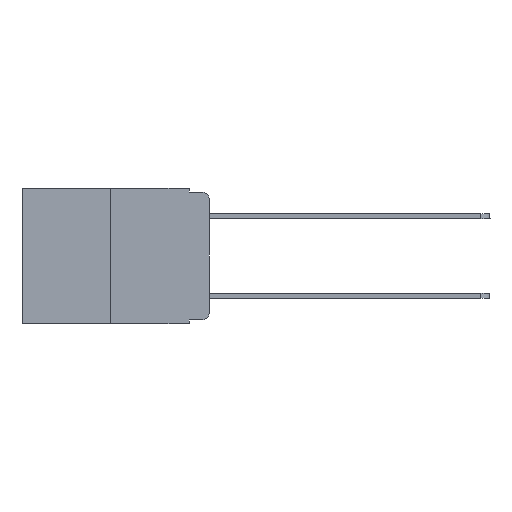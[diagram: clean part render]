
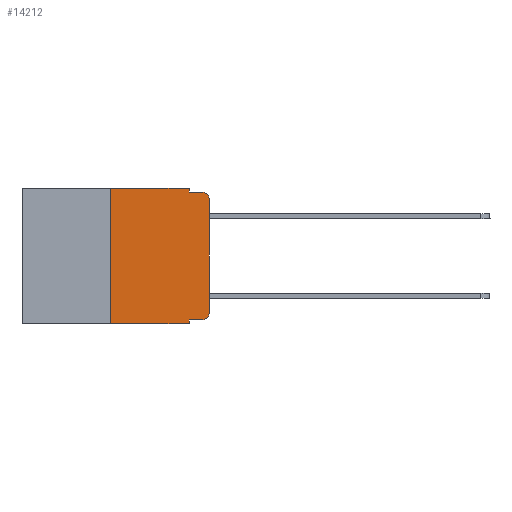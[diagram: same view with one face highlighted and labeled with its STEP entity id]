
A CAD part, left-side view. The second image highlights one B-rep face of the part: STEP entity #14212.
In plain terms, the highlighted planar face has unit normal (-1, 0, 0).
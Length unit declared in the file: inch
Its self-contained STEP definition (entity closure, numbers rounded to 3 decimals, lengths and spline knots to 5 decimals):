
#417 = DIRECTION ( 'NONE',  ( 0., -1., 0. ) ) ;
#524 = CARTESIAN_POINT ( 'NONE',  ( 0., 0.473, -0.343 ) ) ;
#1073 = CARTESIAN_POINT ( 'NONE',  ( 0., 0.051, -0.333 ) ) ;
#1278 = FACE_OUTER_BOUND ( 'NONE', #17155, .T. ) ;
#1283 = LINE ( 'NONE', #1073, #13073 ) ;
#1599 = CARTESIAN_POINT ( 'NONE',  ( 0., 0.051, 0. ) ) ;
#1648 = VECTOR ( 'NONE', #417, 39.37008 ) ;
#1770 = AXIS2_PLACEMENT_3D ( 'NONE', #12779, #19868, #8345 ) ;
#2055 = DIRECTION ( 'NONE',  ( -1., 0., 0. ) ) ;
#2143 = LINE ( 'NONE', #524, #1648 ) ;
#2580 = VERTEX_POINT ( 'NONE', #17380 ) ;
#4154 = CARTESIAN_POINT ( 'NONE',  ( 0., 0.051, 0. ) ) ;
#4368 = ORIENTED_EDGE ( 'NONE', *, *, #5768, .F. ) ;
#4468 = CARTESIAN_POINT ( 'NONE',  ( 0., 0.051, -0.333 ) ) ;
#4494 = CARTESIAN_POINT ( 'NONE',  ( 0., 0.02, -0.01 ) ) ;
#4663 = CARTESIAN_POINT ( 'NONE',  ( 0., 0., -0.03 ) ) ;
#4800 = VECTOR ( 'NONE', #13725, 39.37008 ) ;
#5119 = DIRECTION ( 'NONE',  ( 0., 0., -1. ) ) ;
#5168 = CARTESIAN_POINT ( 'NONE',  ( 0., 0.25, -0.343 ) ) ;
#5503 = CARTESIAN_POINT ( 'NONE',  ( 0., 0.02, -0.313 ) ) ;
#5768 = EDGE_CURVE ( 'NONE', #2580, #7699, #9974, .T. ) ;
#6413 = EDGE_CURVE ( 'NONE', #14480, #19937, #15610, .T. ) ;
#6715 = ORIENTED_EDGE ( 'NONE', *, *, #7337, .F. ) ;
#6822 = ORIENTED_EDGE ( 'NONE', *, *, #6413, .T. ) ;
#6877 = CARTESIAN_POINT ( 'NONE',  ( 0., 0.02, -0.03 ) ) ;
#7066 = AXIS2_PLACEMENT_3D ( 'NONE', #6877, #2055, #11632 ) ;
#7229 = VECTOR ( 'NONE', #16771, 39.37008 ) ;
#7337 = EDGE_CURVE ( 'NONE', #7699, #12888, #12559, .T. ) ;
#7699 = VERTEX_POINT ( 'NONE', #12933 ) ;
#7700 = VECTOR ( 'NONE', #20775, 39.37008 ) ;
#7811 = PLANE ( 'NONE',  #1770 ) ;
#7933 = VERTEX_POINT ( 'NONE', #9357 ) ;
#8112 = DIRECTION ( 'NONE',  ( 0., -1., 0. ) ) ;
#8345 = DIRECTION ( 'NONE',  ( 0., 0., -1. ) ) ;
#9282 = ORIENTED_EDGE ( 'NONE', *, *, #15526, .T. ) ;
#9315 = EDGE_CURVE ( 'NONE', #19937, #12888, #9506, .T. ) ;
#9357 = CARTESIAN_POINT ( 'NONE',  ( 0., 0.051, -0.343 ) ) ;
#9506 = CIRCLE ( 'NONE', #7066, 0.02 ) ;
#9676 = CIRCLE ( 'NONE', #19290, 0.02 ) ;
#9974 = LINE ( 'NONE', #1599, #19733 ) ;
#10031 = VERTEX_POINT ( 'NONE', #12865 ) ;
#10699 = CARTESIAN_POINT ( 'NONE',  ( 0., 0., -0.313 ) ) ;
#10761 = VERTEX_POINT ( 'NONE', #5168 ) ;
#10933 = ORIENTED_EDGE ( 'NONE', *, *, #13773, .F. ) ;
#11137 = EDGE_CURVE ( 'NONE', #10761, #7933, #2143, .T. ) ;
#11632 = DIRECTION ( 'NONE',  ( 0., 0., -1. ) ) ;
#11666 = CARTESIAN_POINT ( 'NONE',  ( 0., 0.25, 0. ) ) ;
#12178 = DIRECTION ( 'NONE',  ( -1., 0., 0. ) ) ;
#12559 = LINE ( 'NONE', #19217, #20457 ) ;
#12779 = CARTESIAN_POINT ( 'NONE',  ( 0., 0.473, 0. ) ) ;
#12865 = CARTESIAN_POINT ( 'NONE',  ( 0., 0.02, -0.333 ) ) ;
#12888 = VERTEX_POINT ( 'NONE', #4494 ) ;
#12933 = CARTESIAN_POINT ( 'NONE',  ( 0., 0.051, -0.01 ) ) ;
#13041 = ORIENTED_EDGE ( 'NONE', *, *, #17055, .F. ) ;
#13052 = LINE ( 'NONE', #11666, #19293 ) ;
#13073 = VECTOR ( 'NONE', #14188, 39.37008 ) ;
#13725 = DIRECTION ( 'NONE',  ( 0., 0., -1. ) ) ;
#13773 = EDGE_CURVE ( 'NONE', #15794, #2580, #14411, .T. ) ;
#14188 = DIRECTION ( 'NONE',  ( 0., -1., 0. ) ) ;
#14212 = ADVANCED_FACE ( 'NONE', ( #1278 ), #7811, .F. ) ;
#14217 = CARTESIAN_POINT ( 'NONE',  ( 0., 0., 0. ) ) ;
#14411 = LINE ( 'NONE', #16344, #7229 ) ;
#14480 = VERTEX_POINT ( 'NONE', #10699 ) ;
#15218 = ORIENTED_EDGE ( 'NONE', *, *, #16032, .F. ) ;
#15356 = ORIENTED_EDGE ( 'NONE', *, *, #9315, .T. ) ;
#15526 = EDGE_CURVE ( 'NONE', #18230, #10031, #1283, .T. ) ;
#15610 = LINE ( 'NONE', #14217, #7700 ) ;
#15794 = VERTEX_POINT ( 'NONE', #19011 ) ;
#15997 = ORIENTED_EDGE ( 'NONE', *, *, #17642, .T. ) ;
#16032 = EDGE_CURVE ( 'NONE', #10761, #15794, #13052, .T. ) ;
#16344 = CARTESIAN_POINT ( 'NONE',  ( 0., 0.473, 0. ) ) ;
#16771 = DIRECTION ( 'NONE',  ( 0., -1., 0. ) ) ;
#17055 = EDGE_CURVE ( 'NONE', #18230, #7933, #17175, .T. ) ;
#17155 = EDGE_LOOP ( 'NONE', ( #6822, #15356, #6715, #4368, #10933, #15218, #19525, #13041, #9282, #15997 ) ) ;
#17175 = LINE ( 'NONE', #4154, #4800 ) ;
#17241 = DIRECTION ( 'NONE',  ( 0., 0., -1. ) ) ;
#17380 = CARTESIAN_POINT ( 'NONE',  ( 0., 0.051, 0. ) ) ;
#17642 = EDGE_CURVE ( 'NONE', #10031, #14480, #9676, .T. ) ;
#18230 = VERTEX_POINT ( 'NONE', #4468 ) ;
#19011 = CARTESIAN_POINT ( 'NONE',  ( 0., 0.25, 0. ) ) ;
#19217 = CARTESIAN_POINT ( 'NONE',  ( 0., 0.051, -0.01 ) ) ;
#19290 = AXIS2_PLACEMENT_3D ( 'NONE', #5503, #12178, #17241 ) ;
#19293 = VECTOR ( 'NONE', #19949, 39.37008 ) ;
#19525 = ORIENTED_EDGE ( 'NONE', *, *, #11137, .T. ) ;
#19733 = VECTOR ( 'NONE', #5119, 39.37008 ) ;
#19868 = DIRECTION ( 'NONE',  ( 1., 0., 0. ) ) ;
#19937 = VERTEX_POINT ( 'NONE', #4663 ) ;
#19949 = DIRECTION ( 'NONE',  ( 0., 0., 1. ) ) ;
#20457 = VECTOR ( 'NONE', #8112, 39.37008 ) ;
#20775 = DIRECTION ( 'NONE',  ( 0., 0., 1. ) ) ;
